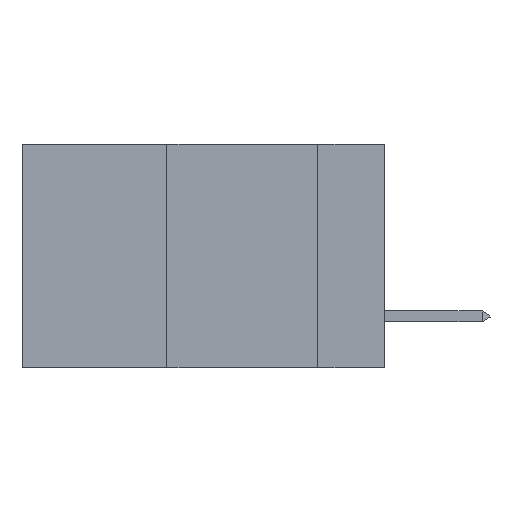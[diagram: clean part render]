
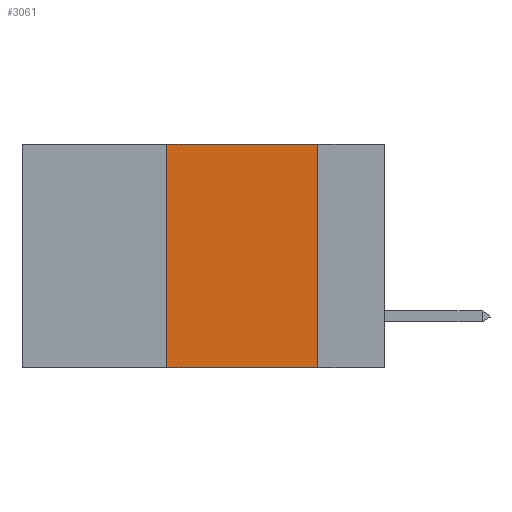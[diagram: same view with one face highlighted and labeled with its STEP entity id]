
A CAD part, left-side view. The second image highlights one B-rep face of the part: STEP entity #3061.
In plain terms, the highlighted planar face has unit normal (-1, 0, 0).
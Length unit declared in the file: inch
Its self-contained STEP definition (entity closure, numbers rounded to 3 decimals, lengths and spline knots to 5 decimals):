
#116 = ORIENTED_EDGE ( 'NONE', *, *, #9975, .T. ) ;
#268 = CARTESIAN_POINT ( 'NONE',  ( 0., 0.6, 0. ) ) ;
#627 = EDGE_LOOP ( 'NONE', ( #9231, #4140, #10534, #116 ) ) ;
#695 = CARTESIAN_POINT ( 'NONE',  ( 0., 0.11, 0. ) ) ;
#868 = AXIS2_PLACEMENT_3D ( 'NONE', #268, #13135, #7869 ) ;
#1155 = VECTOR ( 'NONE', #8306, 39.37008 ) ;
#1360 = CARTESIAN_POINT ( 'NONE',  ( 0., 0.11, -0.37 ) ) ;
#1409 = VERTEX_POINT ( 'NONE', #3729 ) ;
#1850 = LINE ( 'NONE', #3572, #1155 ) ;
#1977 = EDGE_CURVE ( 'NONE', #10059, #4010, #12546, .T. ) ;
#2754 = VERTEX_POINT ( 'NONE', #7861 ) ;
#2925 = FACE_OUTER_BOUND ( 'NONE', #627, .T. ) ;
#3061 = ADVANCED_FACE ( 'NONE', ( #2925 ), #8912, .F. ) ;
#3572 = CARTESIAN_POINT ( 'NONE',  ( 0., 0.36, 0. ) ) ;
#3729 = CARTESIAN_POINT ( 'NONE',  ( 0., 0.36, 0. ) ) ;
#4010 = VERTEX_POINT ( 'NONE', #1360 ) ;
#4140 = ORIENTED_EDGE ( 'NONE', *, *, #8288, .F. ) ;
#4603 = LINE ( 'NONE', #11433, #7124 ) ;
#5422 = CARTESIAN_POINT ( 'NONE',  ( 0., 0.11, 0. ) ) ;
#6898 = EDGE_CURVE ( 'NONE', #2754, #1409, #1850, .T. ) ;
#6983 = VECTOR ( 'NONE', #13287, 39.37008 ) ;
#7124 = VECTOR ( 'NONE', #10384, 39.37008 ) ;
#7494 = VECTOR ( 'NONE', #12405, 39.37008 ) ;
#7861 = CARTESIAN_POINT ( 'NONE',  ( 0., 0.36, -0.37 ) ) ;
#7869 = DIRECTION ( 'NONE',  ( 0., 0., -1. ) ) ;
#8288 = EDGE_CURVE ( 'NONE', #1409, #10059, #10863, .T. ) ;
#8306 = DIRECTION ( 'NONE',  ( 0., 0., 1. ) ) ;
#8880 = CARTESIAN_POINT ( 'NONE',  ( 0., 0.6, 0. ) ) ;
#8912 = PLANE ( 'NONE',  #868 ) ;
#9231 = ORIENTED_EDGE ( 'NONE', *, *, #1977, .F. ) ;
#9975 = EDGE_CURVE ( 'NONE', #2754, #4010, #4603, .T. ) ;
#10059 = VERTEX_POINT ( 'NONE', #5422 ) ;
#10384 = DIRECTION ( 'NONE',  ( 0., -1., 0. ) ) ;
#10534 = ORIENTED_EDGE ( 'NONE', *, *, #6898, .F. ) ;
#10863 = LINE ( 'NONE', #8880, #6983 ) ;
#11433 = CARTESIAN_POINT ( 'NONE',  ( 0., 0.6, -0.37 ) ) ;
#12405 = DIRECTION ( 'NONE',  ( 0., 0., -1. ) ) ;
#12546 = LINE ( 'NONE', #695, #7494 ) ;
#13135 = DIRECTION ( 'NONE',  ( 1., 0., 0. ) ) ;
#13287 = DIRECTION ( 'NONE',  ( 0., -1., 0. ) ) ;
